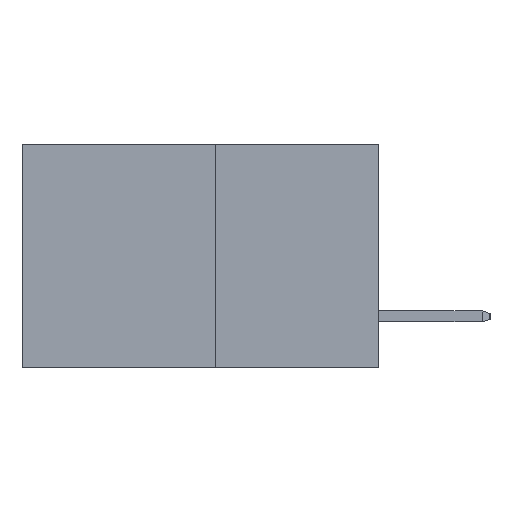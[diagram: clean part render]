
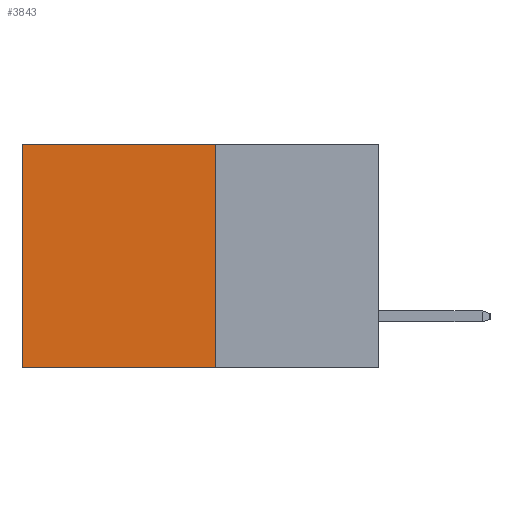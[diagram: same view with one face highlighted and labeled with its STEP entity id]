
A CAD part, left-side view. The second image highlights one B-rep face of the part: STEP entity #3843.
In plain terms, the highlighted planar face has unit normal (-1, 0, 0).
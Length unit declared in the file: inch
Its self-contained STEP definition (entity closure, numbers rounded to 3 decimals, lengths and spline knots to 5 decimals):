
#28 = DIRECTION ( 'NONE',  ( 0., 1., 0. ) ) ;
#975 = FACE_OUTER_BOUND ( 'NONE', #5686, .T. ) ;
#1018 = VERTEX_POINT ( 'NONE', #7162 ) ;
#1940 = LINE ( 'NONE', #8896, #9999 ) ;
#2177 = VECTOR ( 'NONE', #8315, 39.37008 ) ;
#2275 = VERTEX_POINT ( 'NONE', #12610 ) ;
#2480 = EDGE_CURVE ( 'NONE', #8916, #1018, #3166, .T. ) ;
#2520 = CARTESIAN_POINT ( 'NONE',  ( 0.277, 0.27, -0.37 ) ) ;
#3166 = LINE ( 'NONE', #9541, #8642 ) ;
#3843 = ADVANCED_FACE ( 'NONE', ( #975 ), #10016, .F. ) ;
#3913 = EDGE_CURVE ( 'NONE', #2275, #12771, #6166, .T. ) ;
#4602 = ORIENTED_EDGE ( 'NONE', *, *, #7738, .F. ) ;
#5089 = LINE ( 'NONE', #12717, #2177 ) ;
#5520 = ORIENTED_EDGE ( 'NONE', *, *, #3913, .F. ) ;
#5686 = EDGE_LOOP ( 'NONE', ( #9701, #4602, #5520, #5818 ) ) ;
#5818 = ORIENTED_EDGE ( 'NONE', *, *, #10795, .T. ) ;
#6166 = LINE ( 'NONE', #9154, #8740 ) ;
#7162 = CARTESIAN_POINT ( 'NONE',  ( 0.277, 0.59, -0.37 ) ) ;
#7348 = CARTESIAN_POINT ( 'NONE',  ( 0.277, 0.59, 0. ) ) ;
#7738 = EDGE_CURVE ( 'NONE', #12771, #1018, #1940, .T. ) ;
#8315 = DIRECTION ( 'NONE',  ( 0., 1., 0. ) ) ;
#8642 = VECTOR ( 'NONE', #9194, 39.37008 ) ;
#8740 = VECTOR ( 'NONE', #9243, 39.37008 ) ;
#8896 = CARTESIAN_POINT ( 'NONE',  ( 0.277, 0.27, -0.37 ) ) ;
#8916 = VERTEX_POINT ( 'NONE', #7348 ) ;
#9154 = CARTESIAN_POINT ( 'NONE',  ( 0.277, 0.27, -0.37 ) ) ;
#9194 = DIRECTION ( 'NONE',  ( 0., 0., -1. ) ) ;
#9243 = DIRECTION ( 'NONE',  ( 0., 0., -1. ) ) ;
#9541 = CARTESIAN_POINT ( 'NONE',  ( 0.277, 0.59, -0.37 ) ) ;
#9701 = ORIENTED_EDGE ( 'NONE', *, *, #2480, .T. ) ;
#9742 = DIRECTION ( 'NONE',  ( 0., 0., -1. ) ) ;
#9744 = DIRECTION ( 'NONE',  ( 1., 0., 0. ) ) ;
#9988 = CARTESIAN_POINT ( 'NONE',  ( 0.277, 0.27, -0.37 ) ) ;
#9999 = VECTOR ( 'NONE', #28, 39.37008 ) ;
#10016 = PLANE ( 'NONE',  #11812 ) ;
#10795 = EDGE_CURVE ( 'NONE', #2275, #8916, #5089, .T. ) ;
#11812 = AXIS2_PLACEMENT_3D ( 'NONE', #9988, #9744, #9742 ) ;
#12610 = CARTESIAN_POINT ( 'NONE',  ( 0.277, 0.27, 0. ) ) ;
#12717 = CARTESIAN_POINT ( 'NONE',  ( 0.277, 0.27, 0. ) ) ;
#12771 = VERTEX_POINT ( 'NONE', #2520 ) ;
